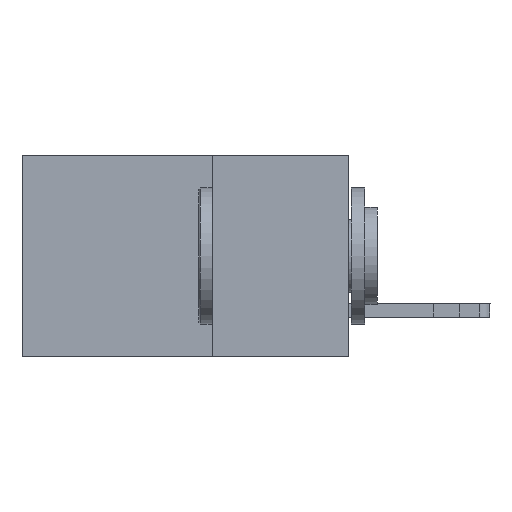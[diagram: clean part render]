
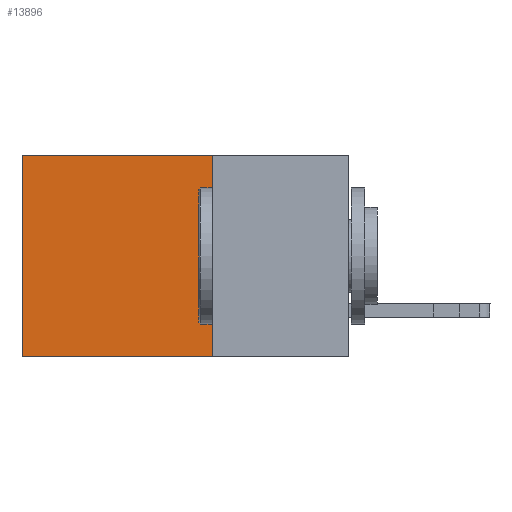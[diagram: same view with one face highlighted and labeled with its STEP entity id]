
A CAD part, left-side view. The second image highlights one B-rep face of the part: STEP entity #13896.
In plain terms, the highlighted planar face has unit normal (-1, 0, 0).
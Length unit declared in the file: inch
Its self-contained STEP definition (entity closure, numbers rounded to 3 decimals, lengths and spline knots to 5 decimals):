
#120 = DIRECTION ( 'NONE',  ( 1., 0., 0. ) ) ;
#178 = DIRECTION ( 'NONE',  ( 0., 0., -1. ) ) ;
#1303 = CARTESIAN_POINT ( 'NONE',  ( 0.2615, 0.6, -0.37 ) ) ;
#1692 = CARTESIAN_POINT ( 'NONE',  ( 0.2615, 0.25, -0.37 ) ) ;
#1747 = LINE ( 'NONE', #5782, #11905 ) ;
#1809 = VECTOR ( 'NONE', #178, 39.37008 ) ;
#3351 = EDGE_CURVE ( 'NONE', #6175, #15240, #1747, .T. ) ;
#3685 = VERTEX_POINT ( 'NONE', #1303 ) ;
#4159 = AXIS2_PLACEMENT_3D ( 'NONE', #14821, #120, #14999 ) ;
#4169 = VECTOR ( 'NONE', #14953, 39.37008 ) ;
#4270 = LINE ( 'NONE', #12110, #4169 ) ;
#5462 = DIRECTION ( 'NONE',  ( 0., 1., 0. ) ) ;
#5782 = CARTESIAN_POINT ( 'NONE',  ( 0.2615, 0.25, 0. ) ) ;
#5984 = ORIENTED_EDGE ( 'NONE', *, *, #3351, .T. ) ;
#6175 = VERTEX_POINT ( 'NONE', #11009 ) ;
#8853 = EDGE_CURVE ( 'NONE', #15346, #3685, #10599, .T. ) ;
#9388 = FACE_OUTER_BOUND ( 'NONE', #11278, .T. ) ;
#10599 = LINE ( 'NONE', #13544, #13441 ) ;
#11009 = CARTESIAN_POINT ( 'NONE',  ( 0.2615, 0.25, 0. ) ) ;
#11118 = ORIENTED_EDGE ( 'NONE', *, *, #12009, .F. ) ;
#11278 = EDGE_LOOP ( 'NONE', ( #11743, #14852, #11118, #5984 ) ) ;
#11743 = ORIENTED_EDGE ( 'NONE', *, *, #14835, .T. ) ;
#11905 = VECTOR ( 'NONE', #16522, 39.37008 ) ;
#12009 = EDGE_CURVE ( 'NONE', #6175, #15346, #12379, .T. ) ;
#12110 = CARTESIAN_POINT ( 'NONE',  ( 0.2615, 0.6, -0.37 ) ) ;
#12379 = LINE ( 'NONE', #1692, #1809 ) ;
#13441 = VECTOR ( 'NONE', #5462, 39.37008 ) ;
#13544 = CARTESIAN_POINT ( 'NONE',  ( 0.2615, 0.25, -0.37 ) ) ;
#13896 = ADVANCED_FACE ( 'NONE', ( #9388 ), #14734, .F. ) ;
#14734 = PLANE ( 'NONE',  #4159 ) ;
#14821 = CARTESIAN_POINT ( 'NONE',  ( 0.2615, 0.25, -0.37 ) ) ;
#14835 = EDGE_CURVE ( 'NONE', #15240, #3685, #4270, .T. ) ;
#14852 = ORIENTED_EDGE ( 'NONE', *, *, #8853, .F. ) ;
#14953 = DIRECTION ( 'NONE',  ( 0., 0., -1. ) ) ;
#14999 = DIRECTION ( 'NONE',  ( 0., 0., -1. ) ) ;
#15240 = VERTEX_POINT ( 'NONE', #17407 ) ;
#15346 = VERTEX_POINT ( 'NONE', #17594 ) ;
#16522 = DIRECTION ( 'NONE',  ( 0., 1., 0. ) ) ;
#17407 = CARTESIAN_POINT ( 'NONE',  ( 0.2615, 0.6, 0. ) ) ;
#17594 = CARTESIAN_POINT ( 'NONE',  ( 0.2615, 0.25, -0.37 ) ) ;
